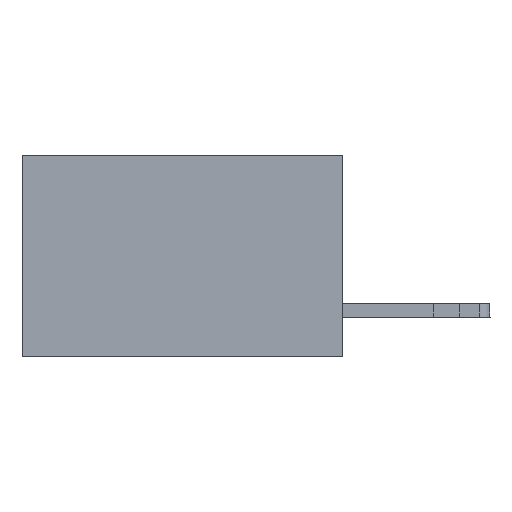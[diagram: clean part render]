
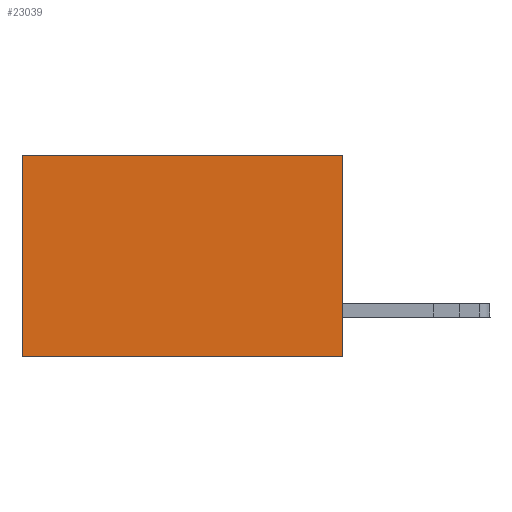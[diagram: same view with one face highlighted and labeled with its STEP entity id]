
A CAD part, left-side view. The second image highlights one B-rep face of the part: STEP entity #23039.
In plain terms, the highlighted planar face has unit normal (-1, 0, 0).
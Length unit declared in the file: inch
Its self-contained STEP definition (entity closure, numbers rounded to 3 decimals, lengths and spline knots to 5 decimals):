
#420 = CARTESIAN_POINT ( 'NONE',  ( 0.277, 0., -0.37 ) ) ;
#1577 = AXIS2_PLACEMENT_3D ( 'NONE', #420, #5704, #15083 ) ;
#2481 = CARTESIAN_POINT ( 'NONE',  ( 0.277, 0.59, -0.37 ) ) ;
#2547 = VERTEX_POINT ( 'NONE', #11318 ) ;
#2563 = EDGE_LOOP ( 'NONE', ( #2647, #5306, #19614, #12520 ) ) ;
#2647 = ORIENTED_EDGE ( 'NONE', *, *, #12923, .T. ) ;
#3132 = LINE ( 'NONE', #12394, #6417 ) ;
#3238 = LINE ( 'NONE', #4677, #15228 ) ;
#4677 = CARTESIAN_POINT ( 'NONE',  ( 0.277, 0., -0.37 ) ) ;
#5306 = ORIENTED_EDGE ( 'NONE', *, *, #14849, .F. ) ;
#5704 = DIRECTION ( 'NONE',  ( 1., 0., 0. ) ) ;
#5984 = VECTOR ( 'NONE', #6351, 39.37008 ) ;
#6351 = DIRECTION ( 'NONE',  ( 0., 1., 0. ) ) ;
#6417 = VECTOR ( 'NONE', #19729, 39.37008 ) ;
#6431 = CARTESIAN_POINT ( 'NONE',  ( 0.277, 0.59, 0. ) ) ;
#6707 = CARTESIAN_POINT ( 'NONE',  ( 0.277, 0., -0.37 ) ) ;
#7721 = CARTESIAN_POINT ( 'NONE',  ( 0.277, 0., 0. ) ) ;
#8504 = LINE ( 'NONE', #6707, #5984 ) ;
#9811 = DIRECTION ( 'NONE',  ( 0., 0., -1. ) ) ;
#11158 = VERTEX_POINT ( 'NONE', #6431 ) ;
#11248 = PLANE ( 'NONE',  #1577 ) ;
#11318 = CARTESIAN_POINT ( 'NONE',  ( 0.277, 0.59, -0.37 ) ) ;
#12394 = CARTESIAN_POINT ( 'NONE',  ( 0.277, 0., 0. ) ) ;
#12520 = ORIENTED_EDGE ( 'NONE', *, *, #19250, .T. ) ;
#12923 = EDGE_CURVE ( 'NONE', #11158, #2547, #18948, .T. ) ;
#14841 = FACE_OUTER_BOUND ( 'NONE', #2563, .T. ) ;
#14849 = EDGE_CURVE ( 'NONE', #20795, #2547, #8504, .T. ) ;
#15083 = DIRECTION ( 'NONE',  ( 0., 0., -1. ) ) ;
#15228 = VECTOR ( 'NONE', #17908, 39.37008 ) ;
#15673 = VERTEX_POINT ( 'NONE', #7721 ) ;
#15772 = EDGE_CURVE ( 'NONE', #15673, #20795, #3238, .T. ) ;
#16910 = CARTESIAN_POINT ( 'NONE',  ( 0.277, 0., -0.37 ) ) ;
#17908 = DIRECTION ( 'NONE',  ( 0., 0., -1. ) ) ;
#18582 = VECTOR ( 'NONE', #9811, 39.37008 ) ;
#18948 = LINE ( 'NONE', #2481, #18582 ) ;
#19250 = EDGE_CURVE ( 'NONE', #15673, #11158, #3132, .T. ) ;
#19614 = ORIENTED_EDGE ( 'NONE', *, *, #15772, .F. ) ;
#19729 = DIRECTION ( 'NONE',  ( 0., 1., 0. ) ) ;
#20795 = VERTEX_POINT ( 'NONE', #16910 ) ;
#23039 = ADVANCED_FACE ( 'NONE', ( #14841 ), #11248, .F. ) ;
